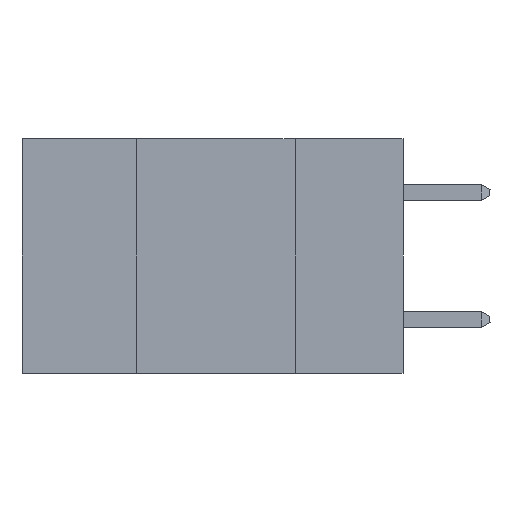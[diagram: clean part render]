
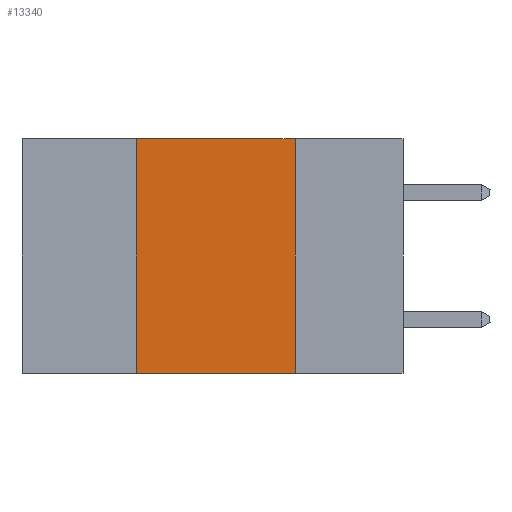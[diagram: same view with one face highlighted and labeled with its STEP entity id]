
A CAD part, left-side view. The second image highlights one B-rep face of the part: STEP entity #13340.
In plain terms, the highlighted planar face has unit normal (-1, 0, 0).
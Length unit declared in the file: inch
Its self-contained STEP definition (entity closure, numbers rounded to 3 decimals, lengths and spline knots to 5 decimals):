
#1957 = CARTESIAN_POINT ( 'NONE',  ( 0., 0.17, -0.37 ) ) ;
#2162 = CARTESIAN_POINT ( 'NONE',  ( 0., 0.6, 0. ) ) ;
#2271 = DIRECTION ( 'NONE',  ( 0., 0., -1. ) ) ;
#3048 = DIRECTION ( 'NONE',  ( 0., -1., 0. ) ) ;
#3246 = ORIENTED_EDGE ( 'NONE', *, *, #19353, .T. ) ;
#4491 = DIRECTION ( 'NONE',  ( 0., 0., -1. ) ) ;
#5122 = AXIS2_PLACEMENT_3D ( 'NONE', #31338, #30998, #2271 ) ;
#5486 = CARTESIAN_POINT ( 'NONE',  ( 0., 0.42, -0.37 ) ) ;
#6720 = VERTEX_POINT ( 'NONE', #1957 ) ;
#6781 = CARTESIAN_POINT ( 'NONE',  ( 0., 0.17, 0. ) ) ;
#6926 = VERTEX_POINT ( 'NONE', #5486 ) ;
#7643 = CARTESIAN_POINT ( 'NONE',  ( 0., 0.42, 0. ) ) ;
#8913 = CARTESIAN_POINT ( 'NONE',  ( 0., 0.42, 0. ) ) ;
#9475 = EDGE_CURVE ( 'NONE', #6926, #11919, #21105, .T. ) ;
#10075 = VECTOR ( 'NONE', #31968, 39.37008 ) ;
#11919 = VERTEX_POINT ( 'NONE', #8913 ) ;
#12752 = VECTOR ( 'NONE', #3048, 39.37008 ) ;
#13340 = ADVANCED_FACE ( 'NONE', ( #13636 ), #30882, .F. ) ;
#13636 = FACE_OUTER_BOUND ( 'NONE', #24920, .T. ) ;
#14934 = ORIENTED_EDGE ( 'NONE', *, *, #9475, .F. ) ;
#15373 = EDGE_CURVE ( 'NONE', #11919, #16062, #18484, .T. ) ;
#16062 = VERTEX_POINT ( 'NONE', #6781 ) ;
#16294 = ORIENTED_EDGE ( 'NONE', *, *, #15373, .F. ) ;
#18484 = LINE ( 'NONE', #2162, #12752 ) ;
#19353 = EDGE_CURVE ( 'NONE', #6926, #6720, #32995, .T. ) ;
#19971 = ORIENTED_EDGE ( 'NONE', *, *, #29085, .F. ) ;
#21105 = LINE ( 'NONE', #7643, #10075 ) ;
#22644 = CARTESIAN_POINT ( 'NONE',  ( 0., 0.17, 0. ) ) ;
#24259 = VECTOR ( 'NONE', #4491, 39.37008 ) ;
#24651 = CARTESIAN_POINT ( 'NONE',  ( 0., 0.6, -0.37 ) ) ;
#24920 = EDGE_LOOP ( 'NONE', ( #19971, #16294, #14934, #3246 ) ) ;
#26887 = VECTOR ( 'NONE', #32691, 39.37008 ) ;
#29085 = EDGE_CURVE ( 'NONE', #16062, #6720, #32777, .T. ) ;
#30882 = PLANE ( 'NONE',  #5122 ) ;
#30998 = DIRECTION ( 'NONE',  ( 1., 0., 0. ) ) ;
#31338 = CARTESIAN_POINT ( 'NONE',  ( 0., 0.6, 0. ) ) ;
#31968 = DIRECTION ( 'NONE',  ( 0., 0., 1. ) ) ;
#32691 = DIRECTION ( 'NONE',  ( 0., -1., 0. ) ) ;
#32777 = LINE ( 'NONE', #22644, #24259 ) ;
#32995 = LINE ( 'NONE', #24651, #26887 ) ;
